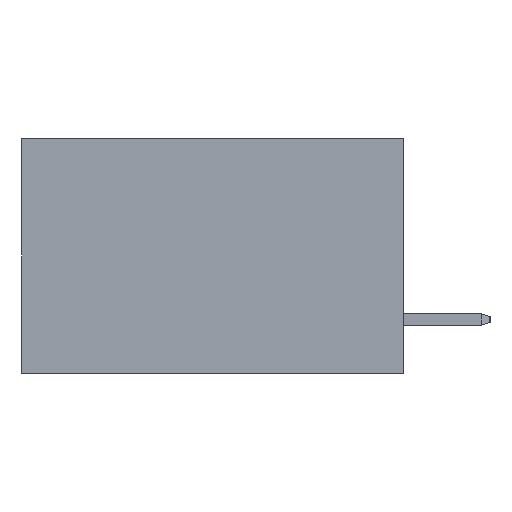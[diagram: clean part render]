
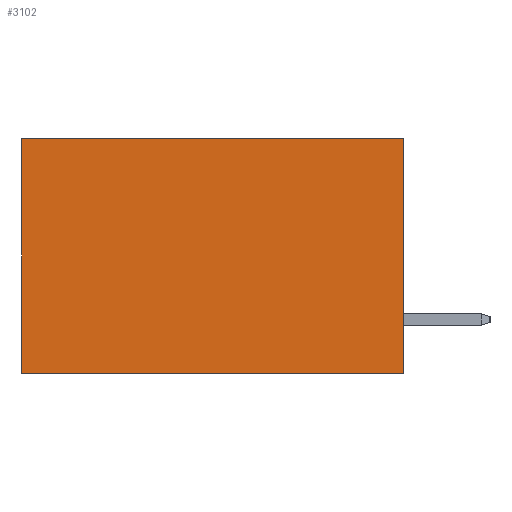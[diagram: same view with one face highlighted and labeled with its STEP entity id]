
A CAD part, left-side view. The second image highlights one B-rep face of the part: STEP entity #3102.
In plain terms, the highlighted planar face has unit normal (-1, 0, 0).
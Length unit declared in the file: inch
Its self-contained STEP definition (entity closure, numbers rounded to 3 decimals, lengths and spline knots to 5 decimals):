
#196 = ORIENTED_EDGE ( 'NONE', *, *, #409, .T. ) ;
#373 = EDGE_LOOP ( 'NONE', ( #196, #3749, #8676, #10123 ) ) ;
#409 = EDGE_CURVE ( 'NONE', #2288, #13931, #11568, .T. ) ;
#972 = CARTESIAN_POINT ( 'NONE',  ( 0.2875, 0., 0. ) ) ;
#2248 = CARTESIAN_POINT ( 'NONE',  ( 0.2875, 0., 0. ) ) ;
#2288 = VERTEX_POINT ( 'NONE', #12348 ) ;
#2697 = DIRECTION ( 'NONE',  ( 0., 1., 0. ) ) ;
#3021 = VECTOR ( 'NONE', #2697, 39.37008 ) ;
#3102 = ADVANCED_FACE ( 'NONE', ( #7312 ), #3533, .F. ) ;
#3533 = PLANE ( 'NONE',  #7614 ) ;
#3749 = ORIENTED_EDGE ( 'NONE', *, *, #15674, .F. ) ;
#4185 = CARTESIAN_POINT ( 'NONE',  ( 0.2875, 0.6, 0. ) ) ;
#4788 = CARTESIAN_POINT ( 'NONE',  ( 0.2875, 0., 0. ) ) ;
#6751 = EDGE_CURVE ( 'NONE', #13975, #8716, #13143, .T. ) ;
#7312 = FACE_OUTER_BOUND ( 'NONE', #373, .T. ) ;
#7614 = AXIS2_PLACEMENT_3D ( 'NONE', #972, #9670, #8443 ) ;
#7829 = VECTOR ( 'NONE', #15587, 39.37008 ) ;
#8443 = DIRECTION ( 'NONE',  ( 0., 0., -1. ) ) ;
#8676 = ORIENTED_EDGE ( 'NONE', *, *, #6751, .F. ) ;
#8716 = VERTEX_POINT ( 'NONE', #10426 ) ;
#9040 = CARTESIAN_POINT ( 'NONE',  ( 0.2875, 0.6, -0.37 ) ) ;
#9397 = LINE ( 'NONE', #10841, #12965 ) ;
#9573 = EDGE_CURVE ( 'NONE', #13975, #2288, #9397, .T. ) ;
#9670 = DIRECTION ( 'NONE',  ( 1., 0., 0. ) ) ;
#10123 = ORIENTED_EDGE ( 'NONE', *, *, #9573, .T. ) ;
#10426 = CARTESIAN_POINT ( 'NONE',  ( 0.2875, 0., -0.37 ) ) ;
#10492 = DIRECTION ( 'NONE',  ( 0., 0., -1. ) ) ;
#10841 = CARTESIAN_POINT ( 'NONE',  ( 0.2875, 0., 0. ) ) ;
#11328 = LINE ( 'NONE', #12380, #3021 ) ;
#11568 = LINE ( 'NONE', #4185, #7829 ) ;
#12348 = CARTESIAN_POINT ( 'NONE',  ( 0.2875, 0.6, 0. ) ) ;
#12380 = CARTESIAN_POINT ( 'NONE',  ( 0.2875, 0., -0.37 ) ) ;
#12965 = VECTOR ( 'NONE', #15817, 39.37008 ) ;
#13143 = LINE ( 'NONE', #2248, #14970 ) ;
#13931 = VERTEX_POINT ( 'NONE', #9040 ) ;
#13975 = VERTEX_POINT ( 'NONE', #4788 ) ;
#14970 = VECTOR ( 'NONE', #10492, 39.37008 ) ;
#15587 = DIRECTION ( 'NONE',  ( 0., 0., -1. ) ) ;
#15674 = EDGE_CURVE ( 'NONE', #8716, #13931, #11328, .T. ) ;
#15817 = DIRECTION ( 'NONE',  ( 0., 1., 0. ) ) ;
